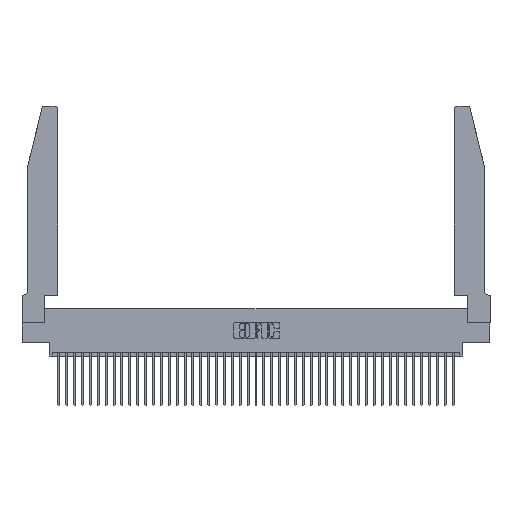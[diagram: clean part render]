
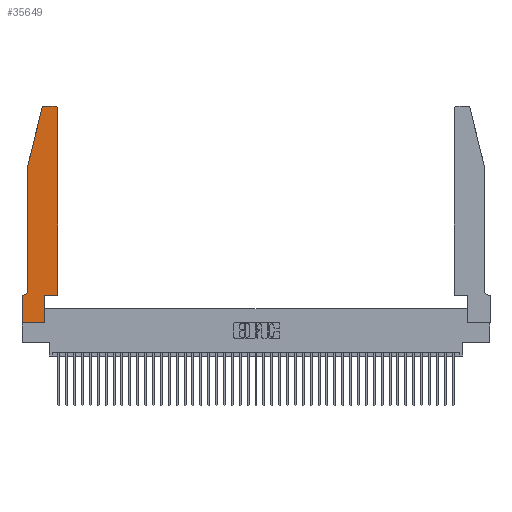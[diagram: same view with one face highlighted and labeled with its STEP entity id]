
A CAD part, top view. The second image highlights one B-rep face of the part: STEP entity #35649.
In plain terms, the highlighted planar face has unit normal (0, 0, 1).
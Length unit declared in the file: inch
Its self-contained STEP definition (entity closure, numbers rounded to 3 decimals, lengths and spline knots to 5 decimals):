
#209 = VERTEX_POINT ( 'NONE', #28623 ) ;
#1052 = EDGE_CURVE ( 'NONE', #37717, #33341, #43558, .T. ) ;
#1351 = CIRCLE ( 'NONE', #6955, 0.03 ) ;
#1584 = CARTESIAN_POINT ( 'NONE',  ( 0.4205, 2.72, 0.37 ) ) ;
#1730 = VECTOR ( 'NONE', #14669, 39.37008 ) ;
#2315 = VERTEX_POINT ( 'NONE', #35279 ) ;
#2584 = VERTEX_POINT ( 'NONE', #33401 ) ;
#5043 = CARTESIAN_POINT ( 'NONE',  ( 0., 0., 0.37 ) ) ;
#5061 = DIRECTION ( 'NONE',  ( 1., 0., 0. ) ) ;
#5196 = ORIENTED_EDGE ( 'NONE', *, *, #13924, .T. ) ;
#5678 = CARTESIAN_POINT ( 'NONE',  ( 0., 0.35, 0.37 ) ) ;
#5806 = ORIENTED_EDGE ( 'NONE', *, *, #21815, .T. ) ;
#6247 = CARTESIAN_POINT ( 'NONE',  ( 0.2865, 0., 0.37 ) ) ;
#6412 = CARTESIAN_POINT ( 'NONE',  ( 0.4505, 0.35, 0.37 ) ) ;
#6955 = AXIS2_PLACEMENT_3D ( 'NONE', #1584, #25412, #5061 ) ;
#8946 = VECTOR ( 'NONE', #34124, 39.37008 ) ;
#8985 = CARTESIAN_POINT ( 'NONE',  ( 0.2865, 0.35, 0.37 ) ) ;
#9154 = DIRECTION ( 'NONE',  ( 0., 0., 1. ) ) ;
#9486 = EDGE_LOOP ( 'NONE', ( #5196, #32931, #14590, #16300, #5806, #13087, #34403, #27960, #11844, #42077, #10832, #16323 ) ) ;
#9827 = LINE ( 'NONE', #34662, #1730 ) ;
#9840 = EDGE_CURVE ( 'NONE', #22758, #19348, #32942, .T. ) ;
#10014 = CARTESIAN_POINT ( 'NONE',  ( 0.4505, 0.35, 0.37 ) ) ;
#10536 = LINE ( 'NONE', #11846, #37299 ) ;
#10659 = VECTOR ( 'NONE', #33557, 39.37008 ) ;
#10832 = ORIENTED_EDGE ( 'NONE', *, *, #13812, .T. ) ;
#11722 = CARTESIAN_POINT ( 'NONE',  ( 0.284, 2.75, 0.37 ) ) ;
#11844 = ORIENTED_EDGE ( 'NONE', *, *, #33506, .T. ) ;
#11846 = CARTESIAN_POINT ( 'NONE',  ( 0., 0., 0.37 ) ) ;
#11880 = VECTOR ( 'NONE', #42476, 39.37008 ) ;
#12003 = DIRECTION ( 'NONE',  ( 0., 0., -1. ) ) ;
#12102 = VERTEX_POINT ( 'NONE', #5043 ) ;
#12595 = CARTESIAN_POINT ( 'NONE',  ( 0.284, 2.72, 0.37 ) ) ;
#13074 = VERTEX_POINT ( 'NONE', #13130 ) ;
#13087 = ORIENTED_EDGE ( 'NONE', *, *, #1052, .T. ) ;
#13130 = CARTESIAN_POINT ( 'NONE',  ( 0.0755, 0.42, 0.37 ) ) ;
#13812 = EDGE_CURVE ( 'NONE', #2584, #209, #35326, .T. ) ;
#13924 = EDGE_CURVE ( 'NONE', #2315, #33378, #30163, .T. ) ;
#14081 = CARTESIAN_POINT ( 'NONE',  ( 0.0755, 2., 0.37 ) ) ;
#14590 = ORIENTED_EDGE ( 'NONE', *, *, #9840, .T. ) ;
#14669 = DIRECTION ( 'NONE',  ( 1., 0., 0. ) ) ;
#15055 = CARTESIAN_POINT ( 'NONE',  ( 0., 0.35, 0.37 ) ) ;
#15855 = CARTESIAN_POINT ( 'NONE',  ( 0.0755, 0.35, 0.37 ) ) ;
#16058 = DIRECTION ( 'NONE',  ( 1., 0., 0. ) ) ;
#16300 = ORIENTED_EDGE ( 'NONE', *, *, #36456, .T. ) ;
#16323 = ORIENTED_EDGE ( 'NONE', *, *, #41126, .T. ) ;
#17075 = CARTESIAN_POINT ( 'NONE',  ( 0.0755, 2., 0.37 ) ) ;
#19348 = VERTEX_POINT ( 'NONE', #41694 ) ;
#19968 = CARTESIAN_POINT ( 'NONE',  ( 0.25487, 2.72718, 0.37 ) ) ;
#21185 = CARTESIAN_POINT ( 'NONE',  ( 0.2605, 2.75, 0.37 ) ) ;
#21815 = EDGE_CURVE ( 'NONE', #13074, #37717, #39176, .T. ) ;
#22045 = VERTEX_POINT ( 'NONE', #6247 ) ;
#22310 = VECTOR ( 'NONE', #27897, 39.37008 ) ;
#22758 = VERTEX_POINT ( 'NONE', #19968 ) ;
#25038 = AXIS2_PLACEMENT_3D ( 'NONE', #5678, #9154, #32716 ) ;
#25412 = DIRECTION ( 'NONE',  ( 0., 0., 1. ) ) ;
#26009 = PLANE ( 'NONE',  #25038 ) ;
#26492 = VECTOR ( 'NONE', #26734, 39.37008 ) ;
#26734 = DIRECTION ( 'NONE',  ( 0., 1., 0. ) ) ;
#27668 = LINE ( 'NONE', #8985, #11880 ) ;
#27897 = DIRECTION ( 'NONE',  ( -1., 0., 0. ) ) ;
#27960 = ORIENTED_EDGE ( 'NONE', *, *, #29955, .T. ) ;
#28623 = CARTESIAN_POINT ( 'NONE',  ( 0.4505, 2.72, 0.37 ) ) ;
#28637 = DIRECTION ( 'NONE',  ( 0., -1., 0. ) ) ;
#29671 = AXIS2_PLACEMENT_3D ( 'NONE', #12595, #36006, #16058 ) ;
#29955 = EDGE_CURVE ( 'NONE', #12102, #22045, #9827, .T. ) ;
#30163 = LINE ( 'NONE', #21185, #22310 ) ;
#31043 = AXIS2_PLACEMENT_3D ( 'NONE', #32134, #12003, #35445 ) ;
#32115 = CIRCLE ( 'NONE', #29671, 0.03 ) ;
#32134 = CARTESIAN_POINT ( 'NONE',  ( 0.0055, 0.42, 0.37 ) ) ;
#32716 = DIRECTION ( 'NONE',  ( 1., 0., 0. ) ) ;
#32931 = ORIENTED_EDGE ( 'NONE', *, *, #41271, .T. ) ;
#32942 = LINE ( 'NONE', #17075, #39704 ) ;
#33341 = VERTEX_POINT ( 'NONE', #15055 ) ;
#33378 = VERTEX_POINT ( 'NONE', #11722 ) ;
#33401 = CARTESIAN_POINT ( 'NONE',  ( 0.4505, 0.35, 0.37 ) ) ;
#33506 = EDGE_CURVE ( 'NONE', #22045, #36693, #27668, .T. ) ;
#33557 = DIRECTION ( 'NONE',  ( 1., 0., 0. ) ) ;
#33730 = CARTESIAN_POINT ( 'NONE',  ( 0.0055, 0.35, 0.37 ) ) ;
#33865 = DIRECTION ( 'NONE',  ( -0.239, -0.971, 0. ) ) ;
#34124 = DIRECTION ( 'NONE',  ( 0., -1., 0. ) ) ;
#34403 = ORIENTED_EDGE ( 'NONE', *, *, #41105, .T. ) ;
#34662 = CARTESIAN_POINT ( 'NONE',  ( 0., 0., 0.37 ) ) ;
#34671 = VECTOR ( 'NONE', #39174, 39.37008 ) ;
#34731 = LINE ( 'NONE', #14081, #8946 ) ;
#35279 = CARTESIAN_POINT ( 'NONE',  ( 0.4205, 2.75, 0.37 ) ) ;
#35326 = LINE ( 'NONE', #6412, #26492 ) ;
#35445 = DIRECTION ( 'NONE',  ( -1., 0., 0. ) ) ;
#35649 = ADVANCED_FACE ( 'NONE', ( #40052 ), #26009, .T. ) ;
#36006 = DIRECTION ( 'NONE',  ( 0., 0., 1. ) ) ;
#36376 = LINE ( 'NONE', #10014, #10659 ) ;
#36456 = EDGE_CURVE ( 'NONE', #19348, #13074, #34731, .T. ) ;
#36693 = VERTEX_POINT ( 'NONE', #41672 ) ;
#37299 = VECTOR ( 'NONE', #28637, 39.37008 ) ;
#37717 = VERTEX_POINT ( 'NONE', #33730 ) ;
#39174 = DIRECTION ( 'NONE',  ( -1., 0., 0. ) ) ;
#39176 = CIRCLE ( 'NONE', #31043, 0.07 ) ;
#39703 = EDGE_CURVE ( 'NONE', #36693, #2584, #36376, .T. ) ;
#39704 = VECTOR ( 'NONE', #33865, 39.37008 ) ;
#40052 = FACE_OUTER_BOUND ( 'NONE', #9486, .T. ) ;
#41105 = EDGE_CURVE ( 'NONE', #33341, #12102, #10536, .T. ) ;
#41126 = EDGE_CURVE ( 'NONE', #209, #2315, #1351, .T. ) ;
#41271 = EDGE_CURVE ( 'NONE', #33378, #22758, #32115, .T. ) ;
#41672 = CARTESIAN_POINT ( 'NONE',  ( 0.2865, 0.35, 0.37 ) ) ;
#41694 = CARTESIAN_POINT ( 'NONE',  ( 0.0755, 2., 0.37 ) ) ;
#42077 = ORIENTED_EDGE ( 'NONE', *, *, #39703, .T. ) ;
#42476 = DIRECTION ( 'NONE',  ( 0., 1., 0. ) ) ;
#43558 = LINE ( 'NONE', #15855, #34671 ) ;
